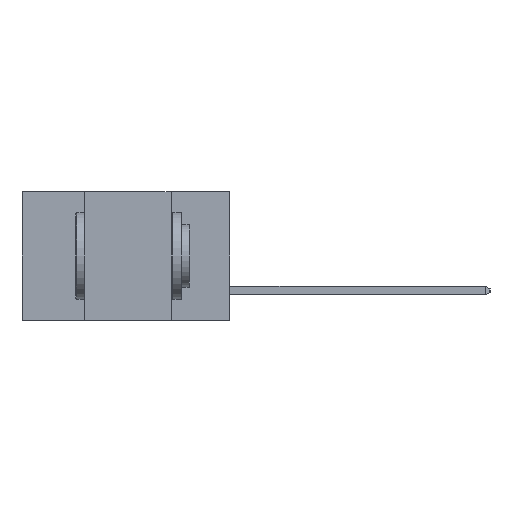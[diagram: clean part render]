
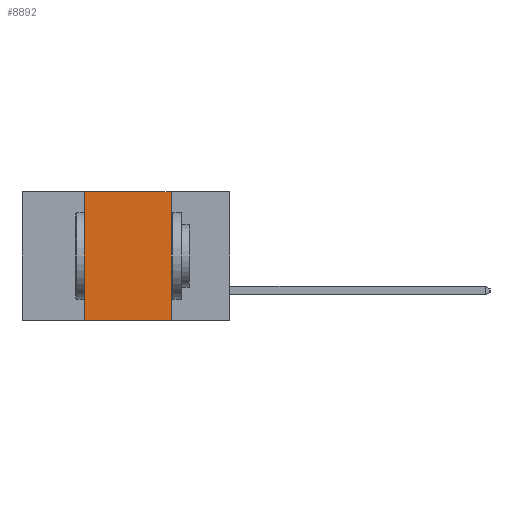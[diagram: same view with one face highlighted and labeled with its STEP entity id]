
A CAD part, left-side view. The second image highlights one B-rep face of the part: STEP entity #8892.
In plain terms, the highlighted planar face has unit normal (-1, 0, 0).
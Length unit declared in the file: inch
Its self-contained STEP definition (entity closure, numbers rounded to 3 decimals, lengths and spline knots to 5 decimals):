
#29 = VECTOR ( 'NONE', #12404, 39.37008 ) ;
#172 = DIRECTION ( 'NONE',  ( 0., 0., 1. ) ) ;
#694 = DIRECTION ( 'NONE',  ( 0., -1., 0. ) ) ;
#1329 = LINE ( 'NONE', #13433, #14149 ) ;
#2475 = FACE_OUTER_BOUND ( 'NONE', #5605, .T. ) ;
#2967 = ORIENTED_EDGE ( 'NONE', *, *, #13041, .F. ) ;
#3321 = DIRECTION ( 'NONE',  ( 0., 0., -1. ) ) ;
#3773 = CARTESIAN_POINT ( 'NONE',  ( 0., 0.17, -0.37 ) ) ;
#3876 = CARTESIAN_POINT ( 'NONE',  ( 0., 0.42, -0.37 ) ) ;
#3898 = LINE ( 'NONE', #4361, #7404 ) ;
#4361 = CARTESIAN_POINT ( 'NONE',  ( 0., 0.6, 0. ) ) ;
#4849 = CARTESIAN_POINT ( 'NONE',  ( 0., 0.17, 0. ) ) ;
#5013 = VERTEX_POINT ( 'NONE', #3876 ) ;
#5424 = VECTOR ( 'NONE', #694, 39.37008 ) ;
#5605 = EDGE_LOOP ( 'NONE', ( #7308, #10161, #2967, #10448 ) ) ;
#5608 = AXIS2_PLACEMENT_3D ( 'NONE', #7255, #11176, #3321 ) ;
#7255 = CARTESIAN_POINT ( 'NONE',  ( 0., 0.6, 0. ) ) ;
#7308 = ORIENTED_EDGE ( 'NONE', *, *, #13921, .F. ) ;
#7335 = CARTESIAN_POINT ( 'NONE',  ( 0., 0.6, -0.37 ) ) ;
#7404 = VECTOR ( 'NONE', #13566, 39.37008 ) ;
#8562 = VERTEX_POINT ( 'NONE', #13240 ) ;
#8892 = ADVANCED_FACE ( 'NONE', ( #2475 ), #16429, .F. ) ;
#9005 = VERTEX_POINT ( 'NONE', #4849 ) ;
#10161 = ORIENTED_EDGE ( 'NONE', *, *, #16136, .F. ) ;
#10384 = EDGE_CURVE ( 'NONE', #5013, #16845, #11943, .T. ) ;
#10448 = ORIENTED_EDGE ( 'NONE', *, *, #10384, .T. ) ;
#10606 = LINE ( 'NONE', #11066, #29 ) ;
#11066 = CARTESIAN_POINT ( 'NONE',  ( 0., 0.17, 0. ) ) ;
#11176 = DIRECTION ( 'NONE',  ( 1., 0., 0. ) ) ;
#11943 = LINE ( 'NONE', #7335, #5424 ) ;
#12404 = DIRECTION ( 'NONE',  ( 0., 0., -1. ) ) ;
#13041 = EDGE_CURVE ( 'NONE', #5013, #8562, #1329, .T. ) ;
#13240 = CARTESIAN_POINT ( 'NONE',  ( 0., 0.42, 0. ) ) ;
#13433 = CARTESIAN_POINT ( 'NONE',  ( 0., 0.42, 0. ) ) ;
#13566 = DIRECTION ( 'NONE',  ( 0., -1., 0. ) ) ;
#13921 = EDGE_CURVE ( 'NONE', #9005, #16845, #10606, .T. ) ;
#14149 = VECTOR ( 'NONE', #172, 39.37008 ) ;
#16136 = EDGE_CURVE ( 'NONE', #8562, #9005, #3898, .T. ) ;
#16429 = PLANE ( 'NONE',  #5608 ) ;
#16845 = VERTEX_POINT ( 'NONE', #3773 ) ;
